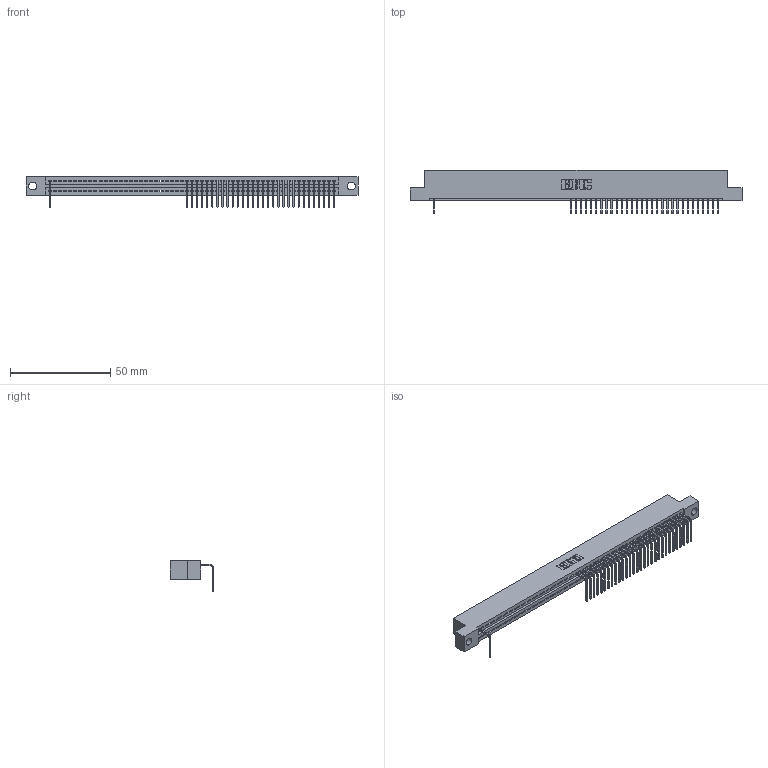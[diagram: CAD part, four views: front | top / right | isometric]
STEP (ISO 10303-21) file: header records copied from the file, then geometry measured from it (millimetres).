
FILE_DESCRIPTION (( 'STEP AP203' ), '1' );
FILE_NAME ('345-057-558-104.STEP', '2018-09-21T11:40:09', ( '' ), ( '' ), 'SwSTEP 2.0', 'SolidWorks 2016', '' );
FILE_SCHEMA (( 'CONFIG_CONTROL_DESIGN' ));
Length unit declared in the file: inch
Products named in the file (3): 345 Part_Flush Mounting Lugs - 0.156 Dia-TH; 345-292-001_558 Tail - 2; 345-057-558-104
Assembly tree (32 placements, depth 2):
  345-057-558-104
    345 Part_Flush Mounting Lugs - 0.156 Dia-TH
    345-292-001_558 Tail - 2  x31
Bounding box: 165.99 x 21.83 x 15.37 mm (x, y, z)
Volume: 15606.4 mm3; surface area: 19778 mm2
Topology: 32 solids, 32 shells, 2402 faces, 7387 edges, 4882 vertices
Faces by surface type: plane 1746, cylinder 656
Entity records: 40135 total; most frequent: ORIENTED_EDGE 7094, CARTESIAN_POINT 7077, DIRECTION 6129, EDGE_CURVE 3547, LINE 3187, VECTOR 3187, VERTEX_POINT 2362, AXIS2_PLACEMENT_3D 1471
